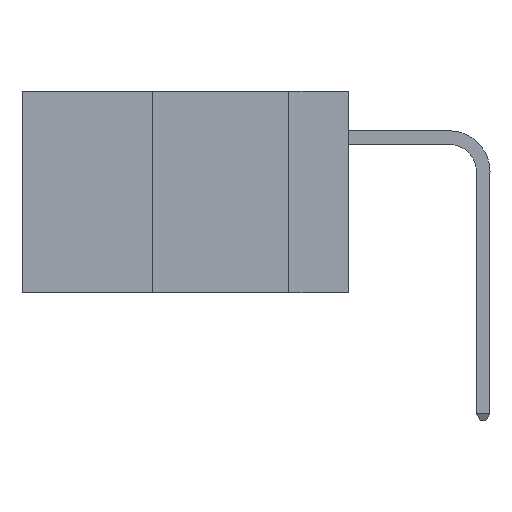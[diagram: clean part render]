
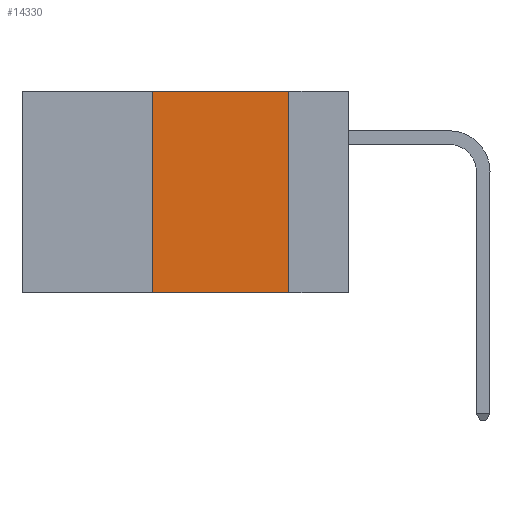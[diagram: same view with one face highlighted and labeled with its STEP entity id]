
A CAD part, left-side view. The second image highlights one B-rep face of the part: STEP entity #14330.
In plain terms, the highlighted planar face has unit normal (-1, 0, 0).
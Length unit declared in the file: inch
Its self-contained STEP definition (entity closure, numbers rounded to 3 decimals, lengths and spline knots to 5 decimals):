
#28 = CARTESIAN_POINT ( 'NONE',  ( 0., 0.11, 0. ) ) ;
#69 = VECTOR ( 'NONE', #4153, 39.37008 ) ;
#92 = CARTESIAN_POINT ( 'NONE',  ( 0., 0.36, 0. ) ) ;
#220 = CARTESIAN_POINT ( 'NONE',  ( 0., 0.36, -0.37 ) ) ;
#1190 = DIRECTION ( 'NONE',  ( 0., -1., 0. ) ) ;
#2384 = ORIENTED_EDGE ( 'NONE', *, *, #13852, .F. ) ;
#2775 = VECTOR ( 'NONE', #1190, 39.37008 ) ;
#2784 = PLANE ( 'NONE',  #4898 ) ;
#3335 = DIRECTION ( 'NONE',  ( 0., 0., 1. ) ) ;
#3793 = LINE ( 'NONE', #20218, #2775 ) ;
#4153 = DIRECTION ( 'NONE',  ( 0., 0., -1. ) ) ;
#4404 = DIRECTION ( 'NONE',  ( 0., 0., -1. ) ) ;
#4898 = AXIS2_PLACEMENT_3D ( 'NONE', #6131, #20525, #4404 ) ;
#5326 = LINE ( 'NONE', #92, #13552 ) ;
#6131 = CARTESIAN_POINT ( 'NONE',  ( 0., 0.6, 0. ) ) ;
#6325 = DIRECTION ( 'NONE',  ( 0., -1., 0. ) ) ;
#6968 = ORIENTED_EDGE ( 'NONE', *, *, #17562, .F. ) ;
#7231 = EDGE_LOOP ( 'NONE', ( #8028, #2384, #6968, #12691 ) ) ;
#7537 = CARTESIAN_POINT ( 'NONE',  ( 0., 0.11, 0. ) ) ;
#8028 = ORIENTED_EDGE ( 'NONE', *, *, #12483, .F. ) ;
#8316 = VERTEX_POINT ( 'NONE', #10754 ) ;
#9627 = CARTESIAN_POINT ( 'NONE',  ( 0., 0.6, -0.37 ) ) ;
#10754 = CARTESIAN_POINT ( 'NONE',  ( 0., 0.36, 0. ) ) ;
#11128 = VERTEX_POINT ( 'NONE', #16034 ) ;
#11948 = FACE_OUTER_BOUND ( 'NONE', #7231, .T. ) ;
#12483 = EDGE_CURVE ( 'NONE', #14966, #11128, #17762, .T. ) ;
#12691 = ORIENTED_EDGE ( 'NONE', *, *, #16991, .T. ) ;
#13552 = VECTOR ( 'NONE', #3335, 39.37008 ) ;
#13578 = LINE ( 'NONE', #9627, #16037 ) ;
#13852 = EDGE_CURVE ( 'NONE', #8316, #14966, #3793, .T. ) ;
#14330 = ADVANCED_FACE ( 'NONE', ( #11948 ), #2784, .F. ) ;
#14966 = VERTEX_POINT ( 'NONE', #28 ) ;
#16034 = CARTESIAN_POINT ( 'NONE',  ( 0., 0.11, -0.37 ) ) ;
#16037 = VECTOR ( 'NONE', #6325, 39.37008 ) ;
#16991 = EDGE_CURVE ( 'NONE', #18834, #11128, #13578, .T. ) ;
#17562 = EDGE_CURVE ( 'NONE', #18834, #8316, #5326, .T. ) ;
#17762 = LINE ( 'NONE', #7537, #69 ) ;
#18834 = VERTEX_POINT ( 'NONE', #220 ) ;
#20218 = CARTESIAN_POINT ( 'NONE',  ( 0., 0.6, 0. ) ) ;
#20525 = DIRECTION ( 'NONE',  ( 1., 0., 0. ) ) ;
